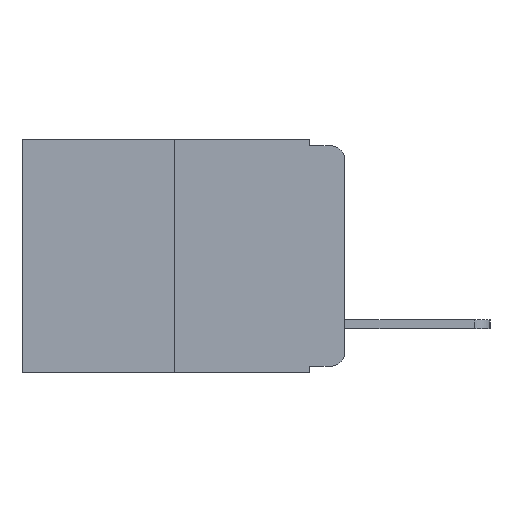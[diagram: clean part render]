
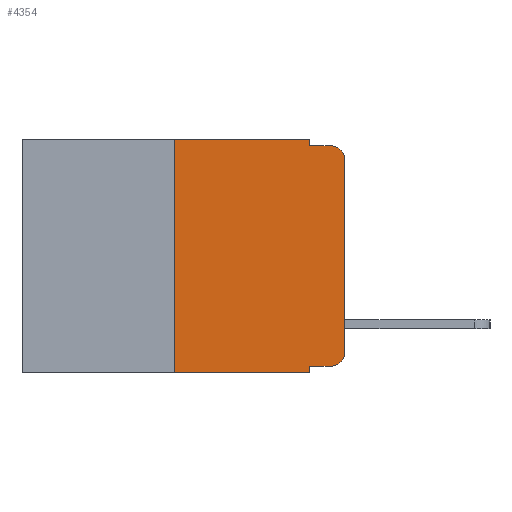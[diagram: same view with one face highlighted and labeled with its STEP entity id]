
A CAD part, left-side view. The second image highlights one B-rep face of the part: STEP entity #4354.
In plain terms, the highlighted planar face has unit normal (-1, 0, 0).
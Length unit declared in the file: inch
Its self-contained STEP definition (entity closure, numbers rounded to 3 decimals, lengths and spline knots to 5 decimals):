
#224 = EDGE_CURVE ( 'NONE', #13907, #5556, #12651, .T. ) ;
#857 = CARTESIAN_POINT ( 'NONE',  ( 0., 0.473, 0. ) ) ;
#914 = VERTEX_POINT ( 'NONE', #6800 ) ;
#1069 = EDGE_LOOP ( 'NONE', ( #9560, #17299, #2209, #10451, #15741, #5186, #13196, #14122, #2472, #12055 ) ) ;
#1124 = EDGE_CURVE ( 'NONE', #4373, #8385, #2608, .T. ) ;
#1126 = CARTESIAN_POINT ( 'NONE',  ( 0., 0.02, -0.313 ) ) ;
#1711 = LINE ( 'NONE', #857, #10902 ) ;
#1852 = LINE ( 'NONE', #15324, #13088 ) ;
#2209 = ORIENTED_EDGE ( 'NONE', *, *, #9126, .F. ) ;
#2472 = ORIENTED_EDGE ( 'NONE', *, *, #15806, .T. ) ;
#2608 = LINE ( 'NONE', #14398, #18108 ) ;
#2737 = DIRECTION ( 'NONE',  ( 0., 0., -1. ) ) ;
#3492 = DIRECTION ( 'NONE',  ( -1., 0., 0. ) ) ;
#3686 = LINE ( 'NONE', #6979, #11367 ) ;
#4119 = LINE ( 'NONE', #17860, #15675 ) ;
#4304 = DIRECTION ( 'NONE',  ( 0., 0., 1. ) ) ;
#4354 = ADVANCED_FACE ( 'NONE', ( #11841 ), #13983, .F. ) ;
#4373 = VERTEX_POINT ( 'NONE', #17439 ) ;
#4693 = CARTESIAN_POINT ( 'NONE',  ( 0., 0.02, -0.01 ) ) ;
#5076 = CIRCLE ( 'NONE', #9867, 0.02 ) ;
#5186 = ORIENTED_EDGE ( 'NONE', *, *, #10511, .F. ) ;
#5556 = VERTEX_POINT ( 'NONE', #18726 ) ;
#5712 = CARTESIAN_POINT ( 'NONE',  ( 0., 0.25, 0. ) ) ;
#5866 = CARTESIAN_POINT ( 'NONE',  ( 0., 0.02, -0.333 ) ) ;
#6311 = VECTOR ( 'NONE', #9573, 39.37008 ) ;
#6800 = CARTESIAN_POINT ( 'NONE',  ( 0., 0.25, -0.343 ) ) ;
#6812 = LINE ( 'NONE', #8069, #6311 ) ;
#6979 = CARTESIAN_POINT ( 'NONE',  ( 0., 0.473, -0.343 ) ) ;
#8005 = DIRECTION ( 'NONE',  ( 0., -1., 0. ) ) ;
#8069 = CARTESIAN_POINT ( 'NONE',  ( 0., 0.051, 0. ) ) ;
#8385 = VERTEX_POINT ( 'NONE', #9659 ) ;
#8782 = CARTESIAN_POINT ( 'NONE',  ( 0., 0.051, -0.01 ) ) ;
#8990 = VERTEX_POINT ( 'NONE', #17927 ) ;
#9045 = AXIS2_PLACEMENT_3D ( 'NONE', #12624, #3492, #14105 ) ;
#9126 = EDGE_CURVE ( 'NONE', #13235, #16580, #1852, .T. ) ;
#9560 = ORIENTED_EDGE ( 'NONE', *, *, #224, .T. ) ;
#9573 = DIRECTION ( 'NONE',  ( 0., 0., -1. ) ) ;
#9659 = CARTESIAN_POINT ( 'NONE',  ( 0., 0.051, -0.343 ) ) ;
#9867 = AXIS2_PLACEMENT_3D ( 'NONE', #1126, #11918, #2737 ) ;
#9898 = EDGE_CURVE ( 'NONE', #17709, #13907, #5076, .T. ) ;
#10088 = EDGE_CURVE ( 'NONE', #8990, #13235, #6812, .T. ) ;
#10451 = ORIENTED_EDGE ( 'NONE', *, *, #10088, .F. ) ;
#10511 = EDGE_CURVE ( 'NONE', #914, #16596, #12146, .T. ) ;
#10833 = AXIS2_PLACEMENT_3D ( 'NONE', #14450, #17651, #18842 ) ;
#10902 = VECTOR ( 'NONE', #17541, 39.37008 ) ;
#11228 = CARTESIAN_POINT ( 'NONE',  ( 0., 0., 0. ) ) ;
#11367 = VECTOR ( 'NONE', #18728, 39.37008 ) ;
#11841 = FACE_OUTER_BOUND ( 'NONE', #1069, .T. ) ;
#11918 = DIRECTION ( 'NONE',  ( -1., 0., 0. ) ) ;
#12055 = ORIENTED_EDGE ( 'NONE', *, *, #9898, .T. ) ;
#12146 = LINE ( 'NONE', #5712, #19439 ) ;
#12624 = CARTESIAN_POINT ( 'NONE',  ( 0., 0.02, -0.03 ) ) ;
#12651 = LINE ( 'NONE', #11228, #16118 ) ;
#13088 = VECTOR ( 'NONE', #8005, 39.37008 ) ;
#13196 = ORIENTED_EDGE ( 'NONE', *, *, #14143, .T. ) ;
#13235 = VERTEX_POINT ( 'NONE', #8782 ) ;
#13518 = DIRECTION ( 'NONE',  ( 0., -1., 0. ) ) ;
#13734 = CARTESIAN_POINT ( 'NONE',  ( 0., 0.25, 0. ) ) ;
#13907 = VERTEX_POINT ( 'NONE', #18227 ) ;
#13983 = PLANE ( 'NONE',  #10833 ) ;
#14010 = EDGE_CURVE ( 'NONE', #5556, #16580, #17991, .T. ) ;
#14105 = DIRECTION ( 'NONE',  ( 0., 0., -1. ) ) ;
#14122 = ORIENTED_EDGE ( 'NONE', *, *, #1124, .F. ) ;
#14143 = EDGE_CURVE ( 'NONE', #914, #8385, #3686, .T. ) ;
#14269 = EDGE_CURVE ( 'NONE', #16596, #8990, #1711, .T. ) ;
#14398 = CARTESIAN_POINT ( 'NONE',  ( 0., 0.051, 0. ) ) ;
#14450 = CARTESIAN_POINT ( 'NONE',  ( 0., 0.473, 0. ) ) ;
#15324 = CARTESIAN_POINT ( 'NONE',  ( 0., 0.051, -0.01 ) ) ;
#15675 = VECTOR ( 'NONE', #13518, 39.37008 ) ;
#15741 = ORIENTED_EDGE ( 'NONE', *, *, #14269, .F. ) ;
#15806 = EDGE_CURVE ( 'NONE', #4373, #17709, #4119, .T. ) ;
#16118 = VECTOR ( 'NONE', #4304, 39.37008 ) ;
#16149 = DIRECTION ( 'NONE',  ( 0., 0., 1. ) ) ;
#16580 = VERTEX_POINT ( 'NONE', #4693 ) ;
#16596 = VERTEX_POINT ( 'NONE', #13734 ) ;
#16832 = DIRECTION ( 'NONE',  ( 0., 0., -1. ) ) ;
#17299 = ORIENTED_EDGE ( 'NONE', *, *, #14010, .T. ) ;
#17439 = CARTESIAN_POINT ( 'NONE',  ( 0., 0.051, -0.333 ) ) ;
#17541 = DIRECTION ( 'NONE',  ( 0., -1., 0. ) ) ;
#17651 = DIRECTION ( 'NONE',  ( 1., 0., 0. ) ) ;
#17709 = VERTEX_POINT ( 'NONE', #5866 ) ;
#17860 = CARTESIAN_POINT ( 'NONE',  ( 0., 0.051, -0.333 ) ) ;
#17927 = CARTESIAN_POINT ( 'NONE',  ( 0., 0.051, 0. ) ) ;
#17991 = CIRCLE ( 'NONE', #9045, 0.02 ) ;
#18108 = VECTOR ( 'NONE', #16832, 39.37008 ) ;
#18227 = CARTESIAN_POINT ( 'NONE',  ( 0., 0., -0.313 ) ) ;
#18726 = CARTESIAN_POINT ( 'NONE',  ( 0., 0., -0.03 ) ) ;
#18728 = DIRECTION ( 'NONE',  ( 0., -1., 0. ) ) ;
#18842 = DIRECTION ( 'NONE',  ( 0., 0., -1. ) ) ;
#19439 = VECTOR ( 'NONE', #16149, 39.37008 ) ;
